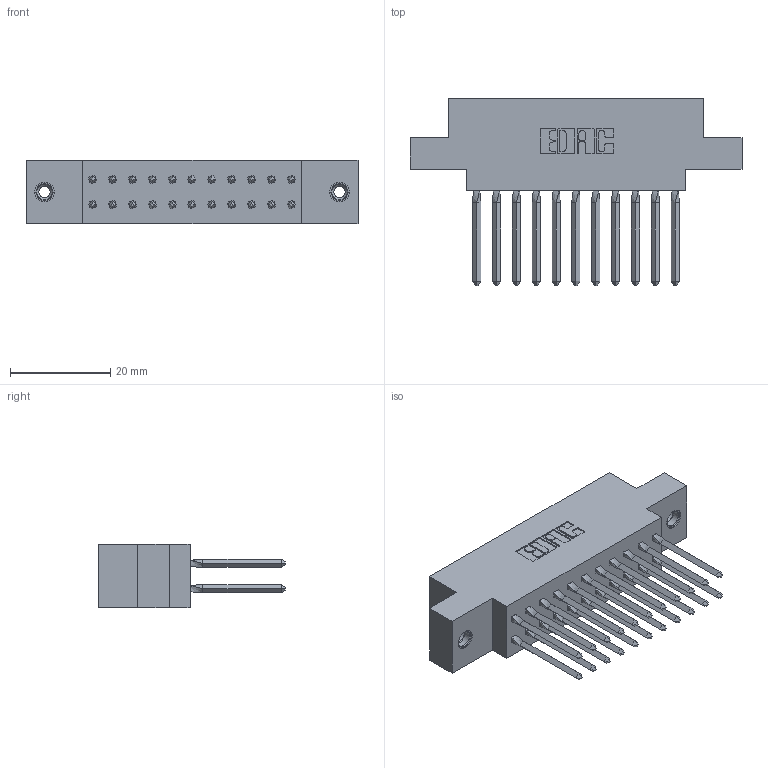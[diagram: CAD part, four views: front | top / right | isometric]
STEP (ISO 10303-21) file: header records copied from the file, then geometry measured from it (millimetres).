
FILE_DESCRIPTION (( 'STEP AP203' ), '1' );
FILE_NAME ('317-022-542-878.STEP', '2020-02-27T17:31:36', ( '' ), ( '' ), 'SwSTEP 2.0', 'SolidWorks 2016', '' );
FILE_SCHEMA (( 'CONFIG_CONTROL_DESIGN' ));
Length unit declared in the file: inch
Products named in the file (4): 345-250-001_345-250-003-102; 317-290-003_542; 317 Part_.156 Dia - TI; 317-022-542-878
Assembly tree (25 placements, depth 2):
  317-022-542-878
    317 Part_.156 Dia - TI
    317-290-003_542  x22
    345-250-001_345-250-003-102  x2
Bounding box: 66.29 x 37.34 x 12.7 mm (x, y, z)
Volume: 9869.2 mm3; surface area: 12751.9 mm2
Topology: 25 solids, 25 shells, 1416 faces, 3931 edges, 2510 vertices
Faces by surface type: plane 1102, cylinder 210, bspline 88, cone 12, torus 4
Entity records: 20428 total; most frequent: CARTESIAN_POINT 3780, ORIENTED_EDGE 3436, DIRECTION 2984, EDGE_CURVE 1718, LINE 1528, VECTOR 1528, VERTEX_POINT 1136, AXIS2_PLACEMENT_3D 728
